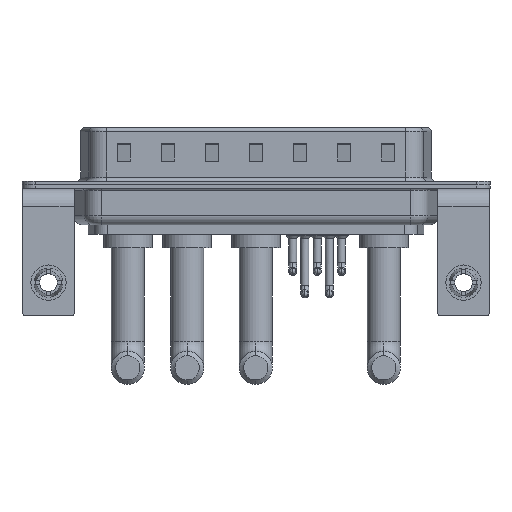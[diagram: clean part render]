
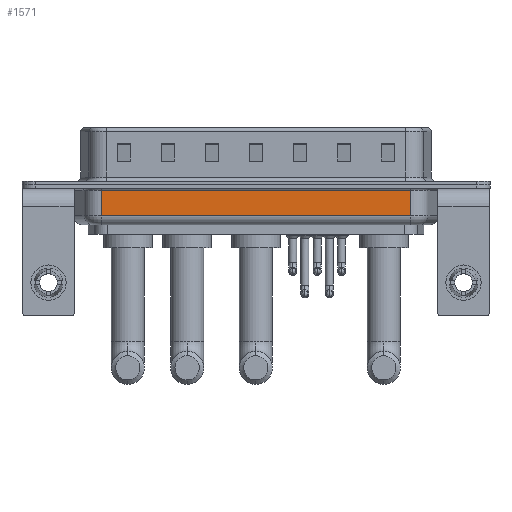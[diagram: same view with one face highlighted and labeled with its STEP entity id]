
A CAD part, front view. The second image highlights one B-rep face of the part: STEP entity #1571.
In plain terms, the highlighted planar face has unit normal (0, -1, 0).
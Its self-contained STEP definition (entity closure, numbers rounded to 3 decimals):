
#1203 = VECTOR ( 'NONE', #1277, 1000. ) ;
#1277 = DIRECTION ( 'NONE',  ( 0., 0., 1. ) ) ;
#1571 = ADVANCED_FACE ( 'NONE', ( #19039 ), #1699, .F. ) ;
#1699 = PLANE ( 'NONE',  #11414 ) ;
#1751 = VERTEX_POINT ( 'NONE', #12446 ) ;
#2565 = DIRECTION ( 'NONE',  ( -1., 0., 0. ) ) ;
#4173 = LINE ( 'NONE', #11900, #6436 ) ;
#4221 = DIRECTION ( 'NONE',  ( 0., 0., 1. ) ) ;
#4341 = CARTESIAN_POINT ( 'NONE',  ( 6.006, -5.35, -0.65 ) ) ;
#5437 = VERTEX_POINT ( 'NONE', #6582 ) ;
#5804 = ORIENTED_EDGE ( 'NONE', *, *, #8520, .T. ) ;
#6135 = DIRECTION ( 'NONE',  ( 0., 0., 1. ) ) ;
#6436 = VECTOR ( 'NONE', #11767, 1000. ) ;
#6582 = CARTESIAN_POINT ( 'NONE',  ( 6.006, -5.35, -0.65 ) ) ;
#6962 = VERTEX_POINT ( 'NONE', #9334 ) ;
#7907 = DIRECTION ( 'NONE',  ( 0., 1., 0. ) ) ;
#8410 = EDGE_CURVE ( 'NONE', #1751, #5437, #21549, .T. ) ;
#8520 = EDGE_CURVE ( 'NONE', #6962, #5437, #16088, .T. ) ;
#8691 = EDGE_CURVE ( 'NONE', #1751, #24173, #4173, .T. ) ;
#8876 = LINE ( 'NONE', #20518, #1203 ) ;
#9275 = ORIENTED_EDGE ( 'NONE', *, *, #9490, .T. ) ;
#9334 = CARTESIAN_POINT ( 'NONE',  ( 41.044, -5.35, -0.65 ) ) ;
#9490 = EDGE_CURVE ( 'NONE', #24173, #6962, #8876, .T. ) ;
#11414 = AXIS2_PLACEMENT_3D ( 'NONE', #24863, #7907, #6135 ) ;
#11767 = DIRECTION ( 'NONE',  ( 1., 0., 0. ) ) ;
#11900 = CARTESIAN_POINT ( 'NONE',  ( 6.006, -5.35, -3.5 ) ) ;
#12446 = CARTESIAN_POINT ( 'NONE',  ( 6.006, -5.35, -3.5 ) ) ;
#12551 = CARTESIAN_POINT ( 'NONE',  ( 41.044, -5.35, -3.5 ) ) ;
#15590 = ORIENTED_EDGE ( 'NONE', *, *, #8691, .T. ) ;
#16088 = LINE ( 'NONE', #4341, #16129 ) ;
#16129 = VECTOR ( 'NONE', #2565, 1000. ) ;
#18146 = VECTOR ( 'NONE', #4221, 1000. ) ;
#19039 = FACE_OUTER_BOUND ( 'NONE', #23108, .T. ) ;
#19150 = CARTESIAN_POINT ( 'NONE',  ( 6.006, -5.35, -4.5 ) ) ;
#20000 = ORIENTED_EDGE ( 'NONE', *, *, #8410, .F. ) ;
#20518 = CARTESIAN_POINT ( 'NONE',  ( 41.044, -5.35, -4.5 ) ) ;
#21549 = LINE ( 'NONE', #19150, #18146 ) ;
#23108 = EDGE_LOOP ( 'NONE', ( #20000, #15590, #9275, #5804 ) ) ;
#24173 = VERTEX_POINT ( 'NONE', #12551 ) ;
#24863 = CARTESIAN_POINT ( 'NONE',  ( 6.006, -5.35, -4.5 ) ) ;
